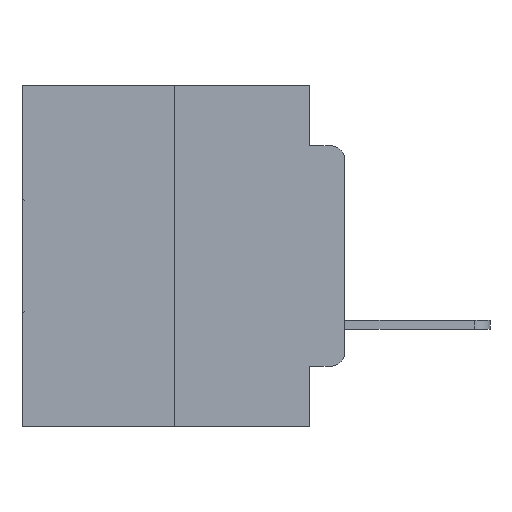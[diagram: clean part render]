
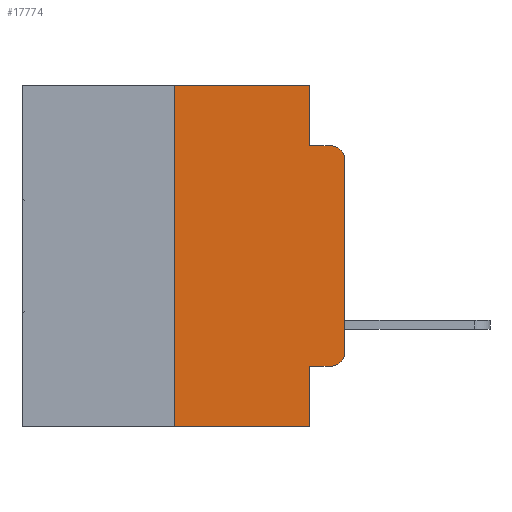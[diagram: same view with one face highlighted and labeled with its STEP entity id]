
A CAD part, left-side view. The second image highlights one B-rep face of the part: STEP entity #17774.
In plain terms, the highlighted planar face has unit normal (-1, 0, 0).
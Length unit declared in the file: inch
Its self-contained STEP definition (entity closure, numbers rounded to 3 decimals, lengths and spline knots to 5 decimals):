
#269 = DIRECTION ( 'NONE',  ( -1., 0., 0. ) ) ;
#313 = VERTEX_POINT ( 'NONE', #1796 ) ;
#1397 = VERTEX_POINT ( 'NONE', #3900 ) ;
#1796 = CARTESIAN_POINT ( 'NONE',  ( 0., 0.051, -0.5 ) ) ;
#2206 = CARTESIAN_POINT ( 'NONE',  ( 0., 0.051, -0.4115 ) ) ;
#2252 = ORIENTED_EDGE ( 'NONE', *, *, #29410, .F. ) ;
#2384 = VECTOR ( 'NONE', #13882, 39.37008 ) ;
#3260 = EDGE_CURVE ( 'NONE', #1397, #9762, #25748, .T. ) ;
#3409 = ORIENTED_EDGE ( 'NONE', *, *, #25210, .F. ) ;
#3900 = CARTESIAN_POINT ( 'NONE',  ( 0., 0., -0.1085 ) ) ;
#6662 = VECTOR ( 'NONE', #7144, 39.37008 ) ;
#6678 = CARTESIAN_POINT ( 'NONE',  ( 0., 0.051, 0. ) ) ;
#6912 = ORIENTED_EDGE ( 'NONE', *, *, #27453, .T. ) ;
#6933 = CARTESIAN_POINT ( 'NONE',  ( 0., 0.051, -0.4115 ) ) ;
#7144 = DIRECTION ( 'NONE',  ( 0., -1., 0. ) ) ;
#7360 = CARTESIAN_POINT ( 'NONE',  ( 0., 0.473, 0. ) ) ;
#7960 = CARTESIAN_POINT ( 'NONE',  ( 0., 0.25, -0.5 ) ) ;
#8146 = AXIS2_PLACEMENT_3D ( 'NONE', #13265, #29151, #15586 ) ;
#8623 = CIRCLE ( 'NONE', #22671, 0.02 ) ;
#8975 = VECTOR ( 'NONE', #14103, 39.37008 ) ;
#9195 = LINE ( 'NONE', #12715, #20898 ) ;
#9267 = DIRECTION ( 'NONE',  ( 0., 0., -1. ) ) ;
#9539 = DIRECTION ( 'NONE',  ( 0., 0., -1. ) ) ;
#9762 = VERTEX_POINT ( 'NONE', #9799 ) ;
#9799 = CARTESIAN_POINT ( 'NONE',  ( 0., 0.02, -0.0885 ) ) ;
#9852 = DIRECTION ( 'NONE',  ( 1., 0., 0. ) ) ;
#10638 = LINE ( 'NONE', #16655, #28199 ) ;
#10690 = VERTEX_POINT ( 'NONE', #7960 ) ;
#11525 = CARTESIAN_POINT ( 'NONE',  ( 0., 0.473, -0.5 ) ) ;
#12040 = CARTESIAN_POINT ( 'NONE',  ( 0., 0.473, 0. ) ) ;
#12263 = EDGE_CURVE ( 'NONE', #28195, #313, #25230, .T. ) ;
#12321 = EDGE_CURVE ( 'NONE', #25634, #9762, #24521, .T. ) ;
#12715 = CARTESIAN_POINT ( 'NONE',  ( 0., 0.25, 0. ) ) ;
#13265 = CARTESIAN_POINT ( 'NONE',  ( 0., 0.02, -0.1085 ) ) ;
#13882 = DIRECTION ( 'NONE',  ( 0., -1., 0. ) ) ;
#14029 = AXIS2_PLACEMENT_3D ( 'NONE', #7360, #9852, #26008 ) ;
#14103 = DIRECTION ( 'NONE',  ( 0., -1., 0. ) ) ;
#14197 = CARTESIAN_POINT ( 'NONE',  ( 0., 0., -0.3915 ) ) ;
#14457 = LINE ( 'NONE', #26284, #19866 ) ;
#14489 = VERTEX_POINT ( 'NONE', #17469 ) ;
#14917 = CARTESIAN_POINT ( 'NONE',  ( 0., 0.02, -0.3915 ) ) ;
#15270 = LINE ( 'NONE', #11525, #2384 ) ;
#15477 = ORIENTED_EDGE ( 'NONE', *, *, #17028, .T. ) ;
#15586 = DIRECTION ( 'NONE',  ( 0., 0., -1. ) ) ;
#16025 = LINE ( 'NONE', #6933, #8975 ) ;
#16541 = VERTEX_POINT ( 'NONE', #20054 ) ;
#16655 = CARTESIAN_POINT ( 'NONE',  ( 0., 0.051, 0. ) ) ;
#16834 = VERTEX_POINT ( 'NONE', #14197 ) ;
#17028 = EDGE_CURVE ( 'NONE', #16834, #1397, #14457, .T. ) ;
#17251 = DIRECTION ( 'NONE',  ( 0., 0., -1. ) ) ;
#17469 = CARTESIAN_POINT ( 'NONE',  ( 0., 0.02, -0.4115 ) ) ;
#17749 = VECTOR ( 'NONE', #25669, 39.37008 ) ;
#17774 = ADVANCED_FACE ( 'NONE', ( #23382 ), #21448, .F. ) ;
#17789 = ORIENTED_EDGE ( 'NONE', *, *, #27035, .T. ) ;
#18366 = ORIENTED_EDGE ( 'NONE', *, *, #3260, .T. ) ;
#19190 = VECTOR ( 'NONE', #9267, 39.37008 ) ;
#19602 = DIRECTION ( 'NONE',  ( 0., 0., 1. ) ) ;
#19752 = CARTESIAN_POINT ( 'NONE',  ( 0., 0.25, 0. ) ) ;
#19866 = VECTOR ( 'NONE', #24031, 39.37008 ) ;
#20054 = CARTESIAN_POINT ( 'NONE',  ( 0., 0.051, 0. ) ) ;
#20535 = ORIENTED_EDGE ( 'NONE', *, *, #12321, .F. ) ;
#20898 = VECTOR ( 'NONE', #19602, 39.37008 ) ;
#21448 = PLANE ( 'NONE',  #14029 ) ;
#22671 = AXIS2_PLACEMENT_3D ( 'NONE', #14917, #269, #17251 ) ;
#23382 = FACE_OUTER_BOUND ( 'NONE', #29730, .T. ) ;
#23840 = ORIENTED_EDGE ( 'NONE', *, *, #12263, .F. ) ;
#24031 = DIRECTION ( 'NONE',  ( 0., 0., 1. ) ) ;
#24521 = LINE ( 'NONE', #27872, #17749 ) ;
#25170 = ORIENTED_EDGE ( 'NONE', *, *, #27100, .F. ) ;
#25210 = EDGE_CURVE ( 'NONE', #16541, #25634, #10638, .T. ) ;
#25230 = LINE ( 'NONE', #6678, #19190 ) ;
#25313 = LINE ( 'NONE', #12040, #6662 ) ;
#25634 = VERTEX_POINT ( 'NONE', #29877 ) ;
#25669 = DIRECTION ( 'NONE',  ( 0., -1., 0. ) ) ;
#25748 = CIRCLE ( 'NONE', #8146, 0.02 ) ;
#26008 = DIRECTION ( 'NONE',  ( 0., 0., -1. ) ) ;
#26284 = CARTESIAN_POINT ( 'NONE',  ( 0., 0., 0. ) ) ;
#26484 = EDGE_CURVE ( 'NONE', #14489, #16834, #8623, .T. ) ;
#27035 = EDGE_CURVE ( 'NONE', #28195, #14489, #16025, .T. ) ;
#27100 = EDGE_CURVE ( 'NONE', #28350, #16541, #25313, .T. ) ;
#27361 = ORIENTED_EDGE ( 'NONE', *, *, #26484, .T. ) ;
#27453 = EDGE_CURVE ( 'NONE', #10690, #313, #15270, .T. ) ;
#27872 = CARTESIAN_POINT ( 'NONE',  ( 0., 0.051, -0.0885 ) ) ;
#28195 = VERTEX_POINT ( 'NONE', #2206 ) ;
#28199 = VECTOR ( 'NONE', #9539, 39.37008 ) ;
#28350 = VERTEX_POINT ( 'NONE', #19752 ) ;
#29151 = DIRECTION ( 'NONE',  ( -1., 0., 0. ) ) ;
#29410 = EDGE_CURVE ( 'NONE', #10690, #28350, #9195, .T. ) ;
#29730 = EDGE_LOOP ( 'NONE', ( #15477, #18366, #20535, #3409, #25170, #2252, #6912, #23840, #17789, #27361 ) ) ;
#29877 = CARTESIAN_POINT ( 'NONE',  ( 0., 0.051, -0.0885 ) ) ;
